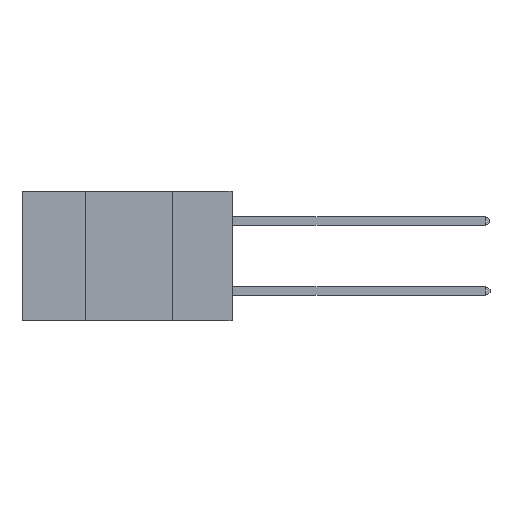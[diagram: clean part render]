
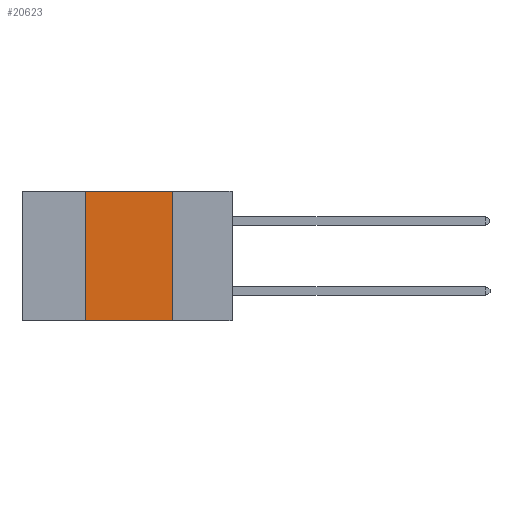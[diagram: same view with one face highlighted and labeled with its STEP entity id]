
A CAD part, left-side view. The second image highlights one B-rep face of the part: STEP entity #20623.
In plain terms, the highlighted planar face has unit normal (-1, 0, 0).
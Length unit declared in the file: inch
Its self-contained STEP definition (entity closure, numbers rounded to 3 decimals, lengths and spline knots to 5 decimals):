
#249 = VERTEX_POINT ( 'NONE', #13965 ) ;
#643 = VECTOR ( 'NONE', #4458, 39.37008 ) ;
#1300 = LINE ( 'NONE', #13500, #643 ) ;
#1469 = CARTESIAN_POINT ( 'NONE',  ( 0., 0.6, 0. ) ) ;
#2546 = AXIS2_PLACEMENT_3D ( 'NONE', #1469, #22806, #12639 ) ;
#4230 = VERTEX_POINT ( 'NONE', #18034 ) ;
#4458 = DIRECTION ( 'NONE',  ( 0., 0., -1. ) ) ;
#4509 = FACE_OUTER_BOUND ( 'NONE', #17880, .T. ) ;
#5067 = EDGE_CURVE ( 'NONE', #5680, #249, #7147, .T. ) ;
#5680 = VERTEX_POINT ( 'NONE', #14281 ) ;
#6418 = EDGE_CURVE ( 'NONE', #249, #4230, #1300, .T. ) ;
#6419 = EDGE_CURVE ( 'NONE', #12877, #5680, #20323, .T. ) ;
#6494 = EDGE_CURVE ( 'NONE', #12877, #4230, #9596, .T. ) ;
#6534 = VECTOR ( 'NONE', #15641, 39.37008 ) ;
#7147 = LINE ( 'NONE', #18696, #6534 ) ;
#9596 = LINE ( 'NONE', #11991, #18725 ) ;
#10938 = ORIENTED_EDGE ( 'NONE', *, *, #6418, .F. ) ;
#11991 = CARTESIAN_POINT ( 'NONE',  ( 0., 0.6, -0.37 ) ) ;
#12003 = ORIENTED_EDGE ( 'NONE', *, *, #6494, .T. ) ;
#12639 = DIRECTION ( 'NONE',  ( 0., 0., -1. ) ) ;
#12877 = VERTEX_POINT ( 'NONE', #13240 ) ;
#13240 = CARTESIAN_POINT ( 'NONE',  ( 0., 0.42, -0.37 ) ) ;
#13500 = CARTESIAN_POINT ( 'NONE',  ( 0., 0.17, 0. ) ) ;
#13702 = DIRECTION ( 'NONE',  ( 0., -1., 0. ) ) ;
#13965 = CARTESIAN_POINT ( 'NONE',  ( 0., 0.17, 0. ) ) ;
#14281 = CARTESIAN_POINT ( 'NONE',  ( 0., 0.42, 0. ) ) ;
#14723 = VECTOR ( 'NONE', #20331, 39.37008 ) ;
#15641 = DIRECTION ( 'NONE',  ( 0., -1., 0. ) ) ;
#17880 = EDGE_LOOP ( 'NONE', ( #10938, #19990, #20532, #12003 ) ) ;
#18034 = CARTESIAN_POINT ( 'NONE',  ( 0., 0.17, -0.37 ) ) ;
#18629 = CARTESIAN_POINT ( 'NONE',  ( 0., 0.42, 0. ) ) ;
#18696 = CARTESIAN_POINT ( 'NONE',  ( 0., 0.6, 0. ) ) ;
#18725 = VECTOR ( 'NONE', #13702, 39.37008 ) ;
#19990 = ORIENTED_EDGE ( 'NONE', *, *, #5067, .F. ) ;
#20323 = LINE ( 'NONE', #18629, #14723 ) ;
#20331 = DIRECTION ( 'NONE',  ( 0., 0., 1. ) ) ;
#20532 = ORIENTED_EDGE ( 'NONE', *, *, #6419, .F. ) ;
#20623 = ADVANCED_FACE ( 'NONE', ( #4509 ), #21124, .F. ) ;
#21124 = PLANE ( 'NONE',  #2546 ) ;
#22806 = DIRECTION ( 'NONE',  ( 1., 0., 0. ) ) ;
